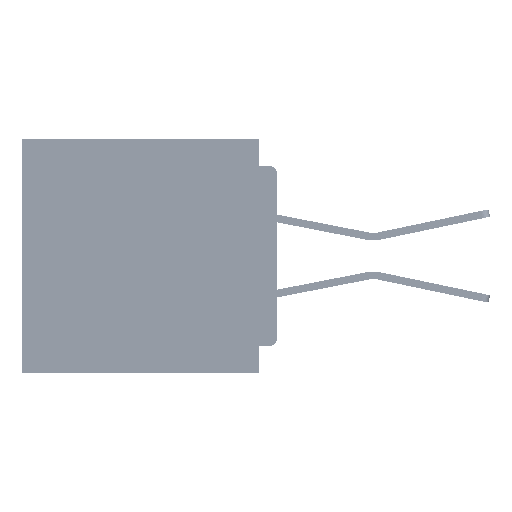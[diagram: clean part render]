
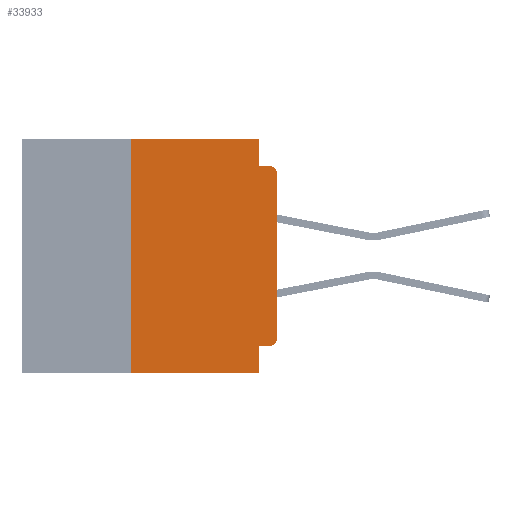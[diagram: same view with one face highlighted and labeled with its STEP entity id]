
A CAD part, left-side view. The second image highlights one B-rep face of the part: STEP entity #33933.
In plain terms, the highlighted planar face has unit normal (-1, 0, 0).
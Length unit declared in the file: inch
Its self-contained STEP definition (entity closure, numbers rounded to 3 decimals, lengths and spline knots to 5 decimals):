
#339 = VECTOR ( 'NONE', #62377, 39.37008 ) ;
#445 = DIRECTION ( 'NONE',  ( 0., -1., 0. ) ) ;
#2093 = ORIENTED_EDGE ( 'NONE', *, *, #40794, .F. ) ;
#2955 = AXIS2_PLACEMENT_3D ( 'NONE', #9777, #46532, #15071 ) ;
#3242 = VERTEX_POINT ( 'NONE', #54712 ) ;
#3892 = AXIS2_PLACEMENT_3D ( 'NONE', #27877, #64612, #33136 ) ;
#4118 = VECTOR ( 'NONE', #56436, 39.37008 ) ;
#4146 = EDGE_CURVE ( 'NONE', #29031, #7932, #21152, .T. ) ;
#6464 = DIRECTION ( 'NONE',  ( 1., 0., 0. ) ) ;
#7498 = DIRECTION ( 'NONE',  ( 0., -1., 0. ) ) ;
#7932 = VERTEX_POINT ( 'NONE', #13652 ) ;
#9777 = CARTESIAN_POINT ( 'NONE',  ( 0., 0.015, -0.06 ) ) ;
#10190 = ORIENTED_EDGE ( 'NONE', *, *, #18281, .T. ) ;
#10542 = ORIENTED_EDGE ( 'NONE', *, *, #4146, .T. ) ;
#12684 = VECTOR ( 'NONE', #445, 39.37008 ) ;
#13111 = VECTOR ( 'NONE', #7498, 39.37008 ) ;
#13652 = CARTESIAN_POINT ( 'NONE',  ( 0., 0.015, -0.045 ) ) ;
#14472 = CARTESIAN_POINT ( 'NONE',  ( 0., 0.031, 0. ) ) ;
#15071 = DIRECTION ( 'NONE',  ( 0., 0., -1. ) ) ;
#15243 = CARTESIAN_POINT ( 'NONE',  ( 0., 0., -0.045 ) ) ;
#15794 = VERTEX_POINT ( 'NONE', #21104 ) ;
#16190 = LINE ( 'NONE', #58468, #40812 ) ;
#16443 = LINE ( 'NONE', #49579, #13111 ) ;
#16628 = DIRECTION ( 'NONE',  ( 0., 0., -1. ) ) ;
#16868 = VERTEX_POINT ( 'NONE', #24651 ) ;
#16873 = CARTESIAN_POINT ( 'NONE',  ( 0., 0.437, 0. ) ) ;
#18136 = ORIENTED_EDGE ( 'NONE', *, *, #42359, .F. ) ;
#18281 = EDGE_CURVE ( 'NONE', #24786, #47153, #29582, .T. ) ;
#19098 = ORIENTED_EDGE ( 'NONE', *, *, #33669, .F. ) ;
#19660 = AXIS2_PLACEMENT_3D ( 'NONE', #16873, #6464, #43232 ) ;
#21104 = CARTESIAN_POINT ( 'NONE',  ( 0., 0.031, -0.355 ) ) ;
#21152 = CIRCLE ( 'NONE', #2955, 0.015 ) ;
#24651 = CARTESIAN_POINT ( 'NONE',  ( 0., 0.25, -0.4 ) ) ;
#24786 = VERTEX_POINT ( 'NONE', #46194 ) ;
#24884 = EDGE_LOOP ( 'NONE', ( #46377, #10542, #51361, #2093, #18136, #37413, #67346, #49310, #19098, #10190 ) ) ;
#27877 = CARTESIAN_POINT ( 'NONE',  ( 0., 0.015, -0.34 ) ) ;
#29031 = VERTEX_POINT ( 'NONE', #45973 ) ;
#29582 = CIRCLE ( 'NONE', #3892, 0.015 ) ;
#30461 = CARTESIAN_POINT ( 'NONE',  ( 0., 0., -0.355 ) ) ;
#32006 = VERTEX_POINT ( 'NONE', #65060 ) ;
#32704 = VECTOR ( 'NONE', #66872, 39.37008 ) ;
#33136 = DIRECTION ( 'NONE',  ( 0., 0., -1. ) ) ;
#33669 = EDGE_CURVE ( 'NONE', #24786, #15794, #47742, .T. ) ;
#33933 = ADVANCED_FACE ( 'NONE', ( #57620 ), #37951, .F. ) ;
#35103 = CARTESIAN_POINT ( 'NONE',  ( 0., 0., 0. ) ) ;
#35228 = LINE ( 'NONE', #35103, #49203 ) ;
#36161 = DIRECTION ( 'NONE',  ( 0., 0., 1. ) ) ;
#37413 = ORIENTED_EDGE ( 'NONE', *, *, #51431, .F. ) ;
#37951 = PLANE ( 'NONE',  #19660 ) ;
#39053 = CARTESIAN_POINT ( 'NONE',  ( 0., 0.031, -0.045 ) ) ;
#40362 = DIRECTION ( 'NONE',  ( 0., 0., 1. ) ) ;
#40794 = EDGE_CURVE ( 'NONE', #40926, #42607, #51662, .T. ) ;
#40812 = VECTOR ( 'NONE', #16628, 39.37008 ) ;
#40926 = VERTEX_POINT ( 'NONE', #47067 ) ;
#42359 = EDGE_CURVE ( 'NONE', #32006, #40926, #53057, .T. ) ;
#42607 = VERTEX_POINT ( 'NONE', #39053 ) ;
#43232 = DIRECTION ( 'NONE',  ( 0., 0., -1. ) ) ;
#43236 = VECTOR ( 'NONE', #36161, 39.37008 ) ;
#45973 = CARTESIAN_POINT ( 'NONE',  ( 0., 0., -0.06 ) ) ;
#46194 = CARTESIAN_POINT ( 'NONE',  ( 0., 0.015, -0.355 ) ) ;
#46377 = ORIENTED_EDGE ( 'NONE', *, *, #64479, .T. ) ;
#46532 = DIRECTION ( 'NONE',  ( -1., 0., 0. ) ) ;
#47067 = CARTESIAN_POINT ( 'NONE',  ( 0., 0.031, 0. ) ) ;
#47153 = VERTEX_POINT ( 'NONE', #57133 ) ;
#47742 = LINE ( 'NONE', #30461, #4118 ) ;
#49069 = EDGE_CURVE ( 'NONE', #42607, #7932, #56363, .T. ) ;
#49203 = VECTOR ( 'NONE', #40362, 39.37008 ) ;
#49310 = ORIENTED_EDGE ( 'NONE', *, *, #65477, .F. ) ;
#49579 = CARTESIAN_POINT ( 'NONE',  ( 0., 0.437, -0.4 ) ) ;
#51361 = ORIENTED_EDGE ( 'NONE', *, *, #49069, .F. ) ;
#51431 = EDGE_CURVE ( 'NONE', #16868, #32006, #57301, .T. ) ;
#51662 = LINE ( 'NONE', #14472, #32704 ) ;
#53057 = LINE ( 'NONE', #63499, #12684 ) ;
#54712 = CARTESIAN_POINT ( 'NONE',  ( 0., 0.031, -0.4 ) ) ;
#56363 = LINE ( 'NONE', #15243, #339 ) ;
#56436 = DIRECTION ( 'NONE',  ( 0., 1., 0. ) ) ;
#57121 = CARTESIAN_POINT ( 'NONE',  ( 0., 0.25, -0.4 ) ) ;
#57133 = CARTESIAN_POINT ( 'NONE',  ( 0., 0., -0.34 ) ) ;
#57301 = LINE ( 'NONE', #57121, #43236 ) ;
#57620 = FACE_OUTER_BOUND ( 'NONE', #24884, .T. ) ;
#58468 = CARTESIAN_POINT ( 'NONE',  ( 0., 0.031, -0.4 ) ) ;
#58478 = EDGE_CURVE ( 'NONE', #16868, #3242, #16443, .T. ) ;
#62377 = DIRECTION ( 'NONE',  ( 0., -1., 0. ) ) ;
#63499 = CARTESIAN_POINT ( 'NONE',  ( 0., 0.437, 0. ) ) ;
#64479 = EDGE_CURVE ( 'NONE', #47153, #29031, #35228, .T. ) ;
#64612 = DIRECTION ( 'NONE',  ( -1., 0., 0. ) ) ;
#65060 = CARTESIAN_POINT ( 'NONE',  ( 0., 0.25, 0. ) ) ;
#65477 = EDGE_CURVE ( 'NONE', #15794, #3242, #16190, .T. ) ;
#66872 = DIRECTION ( 'NONE',  ( 0., 0., -1. ) ) ;
#67346 = ORIENTED_EDGE ( 'NONE', *, *, #58478, .T. ) ;
